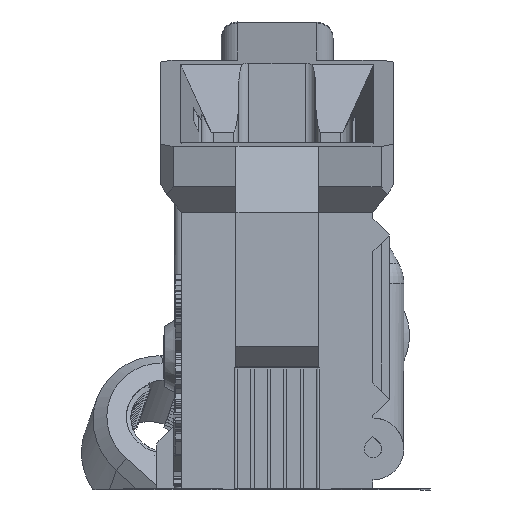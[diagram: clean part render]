
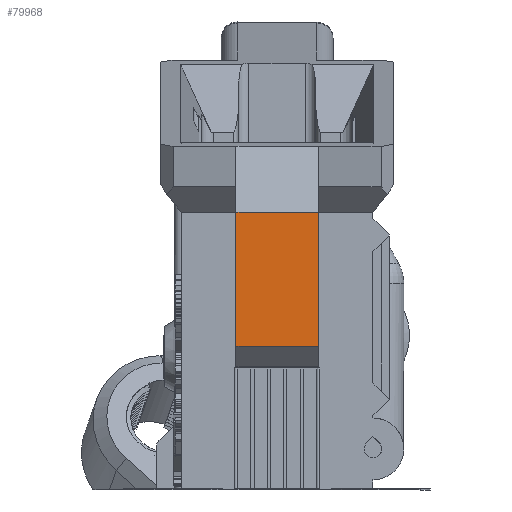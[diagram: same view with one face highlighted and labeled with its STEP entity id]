
A CAD part, left-side view. The second image highlights one B-rep face of the part: STEP entity #79968.
In plain terms, the highlighted planar face has unit normal (-1, 0, 0).
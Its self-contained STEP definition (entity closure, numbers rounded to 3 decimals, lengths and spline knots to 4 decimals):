
#5589 = CARTESIAN_POINT ( 'NONE',  ( -4.187, 0.6526, 1.7032 ) ) ;
#8809 = ORIENTED_EDGE ( 'NONE', *, *, #85344, .F. ) ;
#10191 = VECTOR ( 'NONE', #94167, 39.3701 ) ;
#18701 = ORIENTED_EDGE ( 'NONE', *, *, #116134, .F. ) ;
#26704 = DIRECTION ( 'NONE',  ( 0., 1., 0. ) ) ;
#30239 = EDGE_CURVE ( 'NONE', #81293, #88068, #81413, .T. ) ;
#33221 = CARTESIAN_POINT ( 'NONE',  ( -4.187, 1.1526, 1.7032 ) ) ;
#35751 = CARTESIAN_POINT ( 'NONE',  ( -4.187, -1.0289, 2.518 ) ) ;
#43148 = LINE ( 'NONE', #128569, #147531 ) ;
#48427 = VERTEX_POINT ( 'NONE', #69826 ) ;
#54782 = LINE ( 'NONE', #108471, #62896 ) ;
#55108 = ORIENTED_EDGE ( 'NONE', *, *, #30239, .T. ) ;
#60630 = CARTESIAN_POINT ( 'NONE',  ( -4.187, -1.0289, 1.7032 ) ) ;
#62896 = VECTOR ( 'NONE', #160015, 39.3701 ) ;
#68498 = ORIENTED_EDGE ( 'NONE', *, *, #123969, .T. ) ;
#69826 = CARTESIAN_POINT ( 'NONE',  ( -4.187, 0.6526, 1.7032 ) ) ;
#71783 = AXIS2_PLACEMENT_3D ( 'NONE', #60630, #86408, #112173 ) ;
#77102 = DIRECTION ( 'NONE',  ( 0., 1., 0. ) ) ;
#77264 = VERTEX_POINT ( 'NONE', #33221 ) ;
#77432 = VECTOR ( 'NONE', #26704, 39.3701 ) ;
#79968 = ADVANCED_FACE ( 'NONE', ( #118410 ), #137366, .T. ) ;
#81293 = VERTEX_POINT ( 'NONE', #81465 ) ;
#81413 = LINE ( 'NONE', #35751, #77432 ) ;
#81465 = CARTESIAN_POINT ( 'NONE',  ( -4.187, 0.6526, 2.518 ) ) ;
#85344 = EDGE_CURVE ( 'NONE', #48427, #77264, #43148, .T. ) ;
#86408 = DIRECTION ( 'NONE',  ( -1., 0., 0. ) ) ;
#88068 = VERTEX_POINT ( 'NONE', #104340 ) ;
#94167 = DIRECTION ( 'NONE',  ( 0., 0., 1. ) ) ;
#104340 = CARTESIAN_POINT ( 'NONE',  ( -4.187, 1.1526, 2.518 ) ) ;
#108471 = CARTESIAN_POINT ( 'NONE',  ( -4.187, 1.1526, 2.518 ) ) ;
#112173 = DIRECTION ( 'NONE',  ( 0., 1., 0. ) ) ;
#114607 = LINE ( 'NONE', #5589, #10191 ) ;
#116134 = EDGE_CURVE ( 'NONE', #77264, #88068, #54782, .T. ) ;
#118410 = FACE_OUTER_BOUND ( 'NONE', #139108, .T. ) ;
#123969 = EDGE_CURVE ( 'NONE', #48427, #81293, #114607, .T. ) ;
#128569 = CARTESIAN_POINT ( 'NONE',  ( -4.187, -1.0289, 1.7032 ) ) ;
#137366 = PLANE ( 'NONE',  #71783 ) ;
#139108 = EDGE_LOOP ( 'NONE', ( #68498, #55108, #18701, #8809 ) ) ;
#147531 = VECTOR ( 'NONE', #77102, 39.3701 ) ;
#160015 = DIRECTION ( 'NONE',  ( 0., 0., 1. ) ) ;
